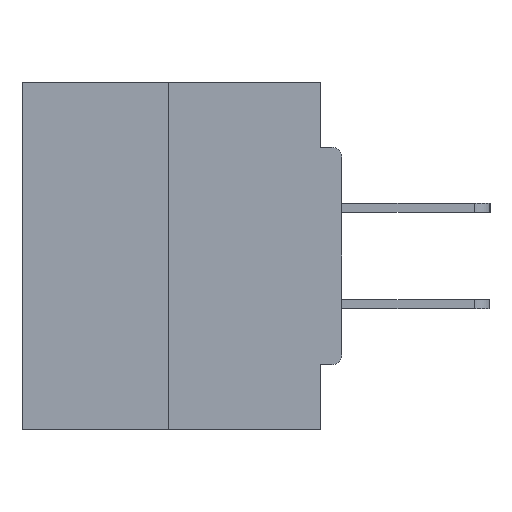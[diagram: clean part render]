
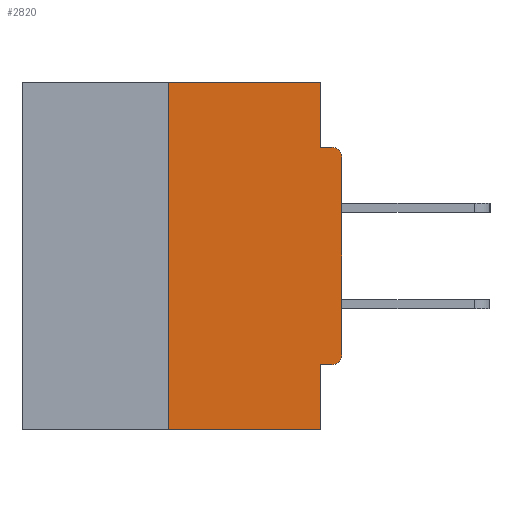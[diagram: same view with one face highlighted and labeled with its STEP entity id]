
A CAD part, left-side view. The second image highlights one B-rep face of the part: STEP entity #2820.
In plain terms, the highlighted planar face has unit normal (-1, 0, 0).
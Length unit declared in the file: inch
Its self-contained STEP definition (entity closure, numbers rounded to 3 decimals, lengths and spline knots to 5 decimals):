
#197 = DIRECTION ( 'NONE',  ( 0., 0., -1. ) ) ;
#788 = CARTESIAN_POINT ( 'NONE',  ( 0., 0.46, 0. ) ) ;
#2010 = CARTESIAN_POINT ( 'NONE',  ( 0., 0., -0.1085 ) ) ;
#2206 = AXIS2_PLACEMENT_3D ( 'NONE', #788, #11099, #13337 ) ;
#2668 = ORIENTED_EDGE ( 'NONE', *, *, #12062, .T. ) ;
#2820 = ADVANCED_FACE ( 'NONE', ( #15990 ), #18632, .F. ) ;
#3019 = LINE ( 'NONE', #19049, #15689 ) ;
#3246 = CARTESIAN_POINT ( 'NONE',  ( 0., 0.25, 0. ) ) ;
#3440 = VECTOR ( 'NONE', #19753, 39.37008 ) ;
#3607 = CARTESIAN_POINT ( 'NONE',  ( 0., 0.015, -0.4065 ) ) ;
#3839 = EDGE_LOOP ( 'NONE', ( #18985, #20769, #20090, #17905, #16609, #11044, #2668, #15909, #4672, #18334 ) ) ;
#4004 = VECTOR ( 'NONE', #29536, 39.37008 ) ;
#4672 = ORIENTED_EDGE ( 'NONE', *, *, #21483, .F. ) ;
#5159 = EDGE_CURVE ( 'NONE', #21584, #32241, #23869, .T. ) ;
#5346 = AXIS2_PLACEMENT_3D ( 'NONE', #32187, #27432, #22107 ) ;
#5671 = VECTOR ( 'NONE', #14191, 39.37008 ) ;
#6124 = AXIS2_PLACEMENT_3D ( 'NONE', #10279, #15377, #197 ) ;
#6141 = VERTEX_POINT ( 'NONE', #31664 ) ;
#6601 = CARTESIAN_POINT ( 'NONE',  ( 0., 0.46, 0. ) ) ;
#8263 = DIRECTION ( 'NONE',  ( 0., -1., 0. ) ) ;
#8696 = VECTOR ( 'NONE', #20256, 39.37008 ) ;
#8743 = DIRECTION ( 'NONE',  ( 0., 0., 1. ) ) ;
#9365 = VERTEX_POINT ( 'NONE', #25810 ) ;
#9491 = EDGE_CURVE ( 'NONE', #19396, #6141, #24755, .T. ) ;
#9654 = VERTEX_POINT ( 'NONE', #24580 ) ;
#10279 = CARTESIAN_POINT ( 'NONE',  ( 0., 0.015, -0.3915 ) ) ;
#11044 = ORIENTED_EDGE ( 'NONE', *, *, #30799, .T. ) ;
#11099 = DIRECTION ( 'NONE',  ( 1., 0., 0. ) ) ;
#11491 = CARTESIAN_POINT ( 'NONE',  ( 0., 0.031, -0.0935 ) ) ;
#11781 = CARTESIAN_POINT ( 'NONE',  ( 0., 0., 0. ) ) ;
#12062 = EDGE_CURVE ( 'NONE', #21180, #24598, #23061, .T. ) ;
#12831 = CARTESIAN_POINT ( 'NONE',  ( 0., 0.031, -0.4065 ) ) ;
#13337 = DIRECTION ( 'NONE',  ( 0., 0., -1. ) ) ;
#13628 = VECTOR ( 'NONE', #14026, 39.37008 ) ;
#14026 = DIRECTION ( 'NONE',  ( 0., -1., 0. ) ) ;
#14191 = DIRECTION ( 'NONE',  ( 0., 0., -1. ) ) ;
#14257 = LINE ( 'NONE', #16109, #21041 ) ;
#14867 = EDGE_CURVE ( 'NONE', #9365, #19396, #3019, .T. ) ;
#15377 = DIRECTION ( 'NONE',  ( -1., 0., 0. ) ) ;
#15689 = VECTOR ( 'NONE', #8743, 39.37008 ) ;
#15909 = ORIENTED_EDGE ( 'NONE', *, *, #21652, .T. ) ;
#15990 = FACE_OUTER_BOUND ( 'NONE', #3839, .T. ) ;
#16109 = CARTESIAN_POINT ( 'NONE',  ( 0., 0., -0.0935 ) ) ;
#16212 = LINE ( 'NONE', #27792, #8696 ) ;
#16609 = ORIENTED_EDGE ( 'NONE', *, *, #5159, .F. ) ;
#17905 = ORIENTED_EDGE ( 'NONE', *, *, #19663, .F. ) ;
#18273 = VECTOR ( 'NONE', #23543, 39.37008 ) ;
#18334 = ORIENTED_EDGE ( 'NONE', *, *, #29458, .F. ) ;
#18632 = PLANE ( 'NONE',  #2206 ) ;
#18985 = ORIENTED_EDGE ( 'NONE', *, *, #9491, .F. ) ;
#19049 = CARTESIAN_POINT ( 'NONE',  ( 0., 0.25, 0. ) ) ;
#19396 = VERTEX_POINT ( 'NONE', #3246 ) ;
#19663 = EDGE_CURVE ( 'NONE', #32241, #9654, #22353, .T. ) ;
#19753 = DIRECTION ( 'NONE',  ( 0., -1., 0. ) ) ;
#20090 = ORIENTED_EDGE ( 'NONE', *, *, #23293, .T. ) ;
#20256 = DIRECTION ( 'NONE',  ( 0., 0., -1. ) ) ;
#20769 = ORIENTED_EDGE ( 'NONE', *, *, #14867, .F. ) ;
#21041 = VECTOR ( 'NONE', #8263, 39.37008 ) ;
#21180 = VERTEX_POINT ( 'NONE', #29794 ) ;
#21483 = EDGE_CURVE ( 'NONE', #32255, #21589, #14257, .T. ) ;
#21584 = VERTEX_POINT ( 'NONE', #3607 ) ;
#21589 = VERTEX_POINT ( 'NONE', #26685 ) ;
#21652 = EDGE_CURVE ( 'NONE', #24598, #21589, #31321, .T. ) ;
#21685 = LINE ( 'NONE', #24527, #3440 ) ;
#22107 = DIRECTION ( 'NONE',  ( 0., 0., -1. ) ) ;
#22353 = LINE ( 'NONE', #29394, #5671 ) ;
#23061 = LINE ( 'NONE', #11781, #4004 ) ;
#23293 = EDGE_CURVE ( 'NONE', #9365, #9654, #21685, .T. ) ;
#23543 = DIRECTION ( 'NONE',  ( 0., 1., 0. ) ) ;
#23712 = CIRCLE ( 'NONE', #6124, 0.015 ) ;
#23869 = LINE ( 'NONE', #31063, #18273 ) ;
#24527 = CARTESIAN_POINT ( 'NONE',  ( 0., 0.46, -0.5 ) ) ;
#24580 = CARTESIAN_POINT ( 'NONE',  ( 0., 0.031, -0.5 ) ) ;
#24598 = VERTEX_POINT ( 'NONE', #2010 ) ;
#24755 = LINE ( 'NONE', #6601, #13628 ) ;
#25810 = CARTESIAN_POINT ( 'NONE',  ( 0., 0.25, -0.5 ) ) ;
#26685 = CARTESIAN_POINT ( 'NONE',  ( 0., 0.015, -0.0935 ) ) ;
#27432 = DIRECTION ( 'NONE',  ( -1., 0., 0. ) ) ;
#27792 = CARTESIAN_POINT ( 'NONE',  ( 0., 0.031, 0. ) ) ;
#29394 = CARTESIAN_POINT ( 'NONE',  ( 0., 0.031, -0.5 ) ) ;
#29458 = EDGE_CURVE ( 'NONE', #6141, #32255, #16212, .T. ) ;
#29536 = DIRECTION ( 'NONE',  ( 0., 0., 1. ) ) ;
#29794 = CARTESIAN_POINT ( 'NONE',  ( 0., 0., -0.3915 ) ) ;
#30799 = EDGE_CURVE ( 'NONE', #21584, #21180, #23712, .T. ) ;
#31063 = CARTESIAN_POINT ( 'NONE',  ( 0., 0., -0.4065 ) ) ;
#31321 = CIRCLE ( 'NONE', #5346, 0.015 ) ;
#31664 = CARTESIAN_POINT ( 'NONE',  ( 0., 0.031, 0. ) ) ;
#32187 = CARTESIAN_POINT ( 'NONE',  ( 0., 0.015, -0.1085 ) ) ;
#32241 = VERTEX_POINT ( 'NONE', #12831 ) ;
#32255 = VERTEX_POINT ( 'NONE', #11491 ) ;
